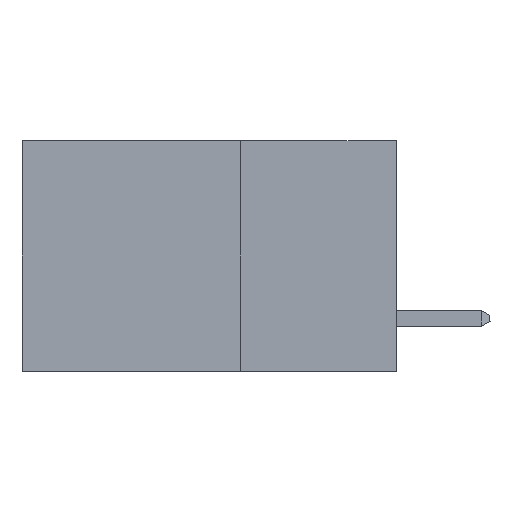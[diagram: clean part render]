
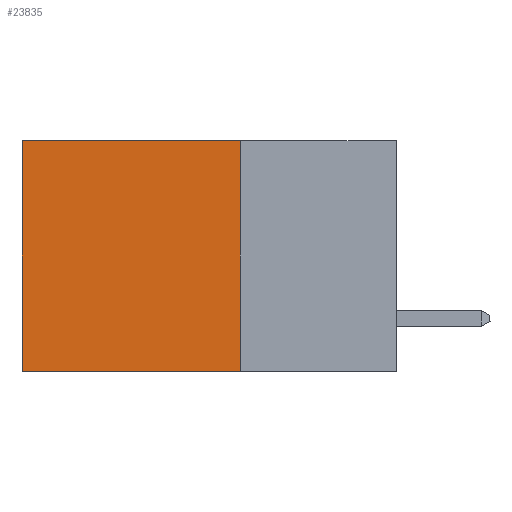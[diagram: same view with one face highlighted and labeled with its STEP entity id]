
A CAD part, left-side view. The second image highlights one B-rep face of the part: STEP entity #23835.
In plain terms, the highlighted planar face has unit normal (-1, 0, 0).
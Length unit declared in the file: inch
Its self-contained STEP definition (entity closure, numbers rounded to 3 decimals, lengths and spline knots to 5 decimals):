
#612 = VECTOR ( 'NONE', #16434, 39.37008 ) ;
#776 = VERTEX_POINT ( 'NONE', #17777 ) ;
#1221 = EDGE_CURVE ( 'NONE', #19992, #2327, #30150, .T. ) ;
#2327 = VERTEX_POINT ( 'NONE', #6416 ) ;
#2784 = DIRECTION ( 'NONE',  ( 1., 0., 0. ) ) ;
#3853 = VERTEX_POINT ( 'NONE', #27180 ) ;
#4008 = ORIENTED_EDGE ( 'NONE', *, *, #24396, .F. ) ;
#4783 = DIRECTION ( 'NONE',  ( 0., 0., -1. ) ) ;
#4818 = LINE ( 'NONE', #11753, #612 ) ;
#6416 = CARTESIAN_POINT ( 'NONE',  ( 0.298, 0.6, -0.37 ) ) ;
#8081 = ORIENTED_EDGE ( 'NONE', *, *, #23307, .T. ) ;
#8626 = VECTOR ( 'NONE', #4783, 39.37008 ) ;
#9927 = FACE_OUTER_BOUND ( 'NONE', #11633, .T. ) ;
#10139 = EDGE_CURVE ( 'NONE', #776, #3853, #10182, .T. ) ;
#10182 = LINE ( 'NONE', #20730, #23205 ) ;
#11633 = EDGE_LOOP ( 'NONE', ( #16056, #4008, #19963, #8081 ) ) ;
#11753 = CARTESIAN_POINT ( 'NONE',  ( 0.298, 0.25, -0.37 ) ) ;
#12668 = CARTESIAN_POINT ( 'NONE',  ( 0.298, 0.25, 0. ) ) ;
#14971 = PLANE ( 'NONE',  #25917 ) ;
#16056 = ORIENTED_EDGE ( 'NONE', *, *, #1221, .T. ) ;
#16434 = DIRECTION ( 'NONE',  ( 0., 1., 0. ) ) ;
#17777 = CARTESIAN_POINT ( 'NONE',  ( 0.298, 0.25, 0. ) ) ;
#18412 = CARTESIAN_POINT ( 'NONE',  ( 0.298, 0.25, 0. ) ) ;
#18719 = DIRECTION ( 'NONE',  ( 0., 1., 0. ) ) ;
#19963 = ORIENTED_EDGE ( 'NONE', *, *, #10139, .F. ) ;
#19992 = VERTEX_POINT ( 'NONE', #24227 ) ;
#20730 = CARTESIAN_POINT ( 'NONE',  ( 0.298, 0.25, 0. ) ) ;
#21431 = LINE ( 'NONE', #18412, #26033 ) ;
#22898 = DIRECTION ( 'NONE',  ( 0., 0., -1. ) ) ;
#23205 = VECTOR ( 'NONE', #22898, 39.37008 ) ;
#23307 = EDGE_CURVE ( 'NONE', #776, #19992, #21431, .T. ) ;
#23835 = ADVANCED_FACE ( 'NONE', ( #9927 ), #14971, .F. ) ;
#24227 = CARTESIAN_POINT ( 'NONE',  ( 0.298, 0.6, 0. ) ) ;
#24396 = EDGE_CURVE ( 'NONE', #3853, #2327, #4818, .T. ) ;
#25917 = AXIS2_PLACEMENT_3D ( 'NONE', #12668, #2784, #27352 ) ;
#26033 = VECTOR ( 'NONE', #18719, 39.37008 ) ;
#26781 = CARTESIAN_POINT ( 'NONE',  ( 0.298, 0.6, 0. ) ) ;
#27180 = CARTESIAN_POINT ( 'NONE',  ( 0.298, 0.25, -0.37 ) ) ;
#27352 = DIRECTION ( 'NONE',  ( 0., 0., -1. ) ) ;
#30150 = LINE ( 'NONE', #26781, #8626 ) ;
